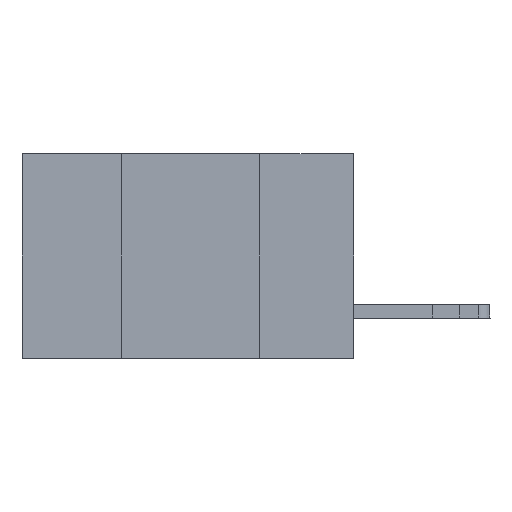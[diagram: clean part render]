
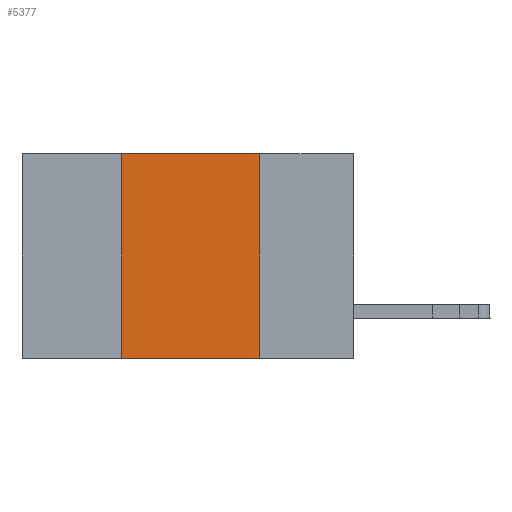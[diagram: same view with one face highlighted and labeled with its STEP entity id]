
A CAD part, left-side view. The second image highlights one B-rep face of the part: STEP entity #5377.
In plain terms, the highlighted planar face has unit normal (-1, 0, 0).
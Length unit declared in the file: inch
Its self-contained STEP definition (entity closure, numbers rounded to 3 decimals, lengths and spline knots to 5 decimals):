
#394 = VERTEX_POINT ( 'NONE', #6386 ) ;
#1948 = DIRECTION ( 'NONE',  ( 0., 0., -1. ) ) ;
#2194 = VERTEX_POINT ( 'NONE', #29420 ) ;
#3750 = CARTESIAN_POINT ( 'NONE',  ( 0., 0.6, -0.37 ) ) ;
#5377 = ADVANCED_FACE ( 'NONE', ( #24459 ), #15068, .F. ) ;
#5872 = VERTEX_POINT ( 'NONE', #25013 ) ;
#6386 = CARTESIAN_POINT ( 'NONE',  ( 0., 0.42, 0. ) ) ;
#6483 = DIRECTION ( 'NONE',  ( 0., -1., 0. ) ) ;
#6911 = DIRECTION ( 'NONE',  ( 1., 0., 0. ) ) ;
#7317 = CARTESIAN_POINT ( 'NONE',  ( 0., 0.17, 0. ) ) ;
#8722 = AXIS2_PLACEMENT_3D ( 'NONE', #23239, #6911, #25847 ) ;
#8817 = DIRECTION ( 'NONE',  ( 0., -1., 0. ) ) ;
#9220 = ORIENTED_EDGE ( 'NONE', *, *, #28491, .F. ) ;
#10951 = ORIENTED_EDGE ( 'NONE', *, *, #16478, .F. ) ;
#15068 = PLANE ( 'NONE',  #8722 ) ;
#15737 = EDGE_LOOP ( 'NONE', ( #9220, #10951, #18213, #32232 ) ) ;
#16478 = EDGE_CURVE ( 'NONE', #394, #24545, #31373, .T. ) ;
#17308 = CARTESIAN_POINT ( 'NONE',  ( 0., 0.17, 0. ) ) ;
#17313 = VECTOR ( 'NONE', #8817, 39.37008 ) ;
#18213 = ORIENTED_EDGE ( 'NONE', *, *, #24857, .F. ) ;
#19241 = VECTOR ( 'NONE', #6483, 39.37008 ) ;
#19705 = CARTESIAN_POINT ( 'NONE',  ( 0., 0.6, 0. ) ) ;
#22468 = VECTOR ( 'NONE', #1948, 39.37008 ) ;
#22738 = VECTOR ( 'NONE', #23661, 39.37008 ) ;
#23239 = CARTESIAN_POINT ( 'NONE',  ( 0., 0.6, 0. ) ) ;
#23661 = DIRECTION ( 'NONE',  ( 0., 0., 1. ) ) ;
#24459 = FACE_OUTER_BOUND ( 'NONE', #15737, .T. ) ;
#24545 = VERTEX_POINT ( 'NONE', #17308 ) ;
#24857 = EDGE_CURVE ( 'NONE', #2194, #394, #29676, .T. ) ;
#25013 = CARTESIAN_POINT ( 'NONE',  ( 0., 0.17, -0.37 ) ) ;
#25847 = DIRECTION ( 'NONE',  ( 0., 0., -1. ) ) ;
#28491 = EDGE_CURVE ( 'NONE', #24545, #5872, #29422, .T. ) ;
#29420 = CARTESIAN_POINT ( 'NONE',  ( 0., 0.42, -0.37 ) ) ;
#29422 = LINE ( 'NONE', #7317, #22468 ) ;
#29676 = LINE ( 'NONE', #31398, #22738 ) ;
#31373 = LINE ( 'NONE', #19705, #17313 ) ;
#31398 = CARTESIAN_POINT ( 'NONE',  ( 0., 0.42, 0. ) ) ;
#31930 = EDGE_CURVE ( 'NONE', #2194, #5872, #34017, .T. ) ;
#32232 = ORIENTED_EDGE ( 'NONE', *, *, #31930, .T. ) ;
#34017 = LINE ( 'NONE', #3750, #19241 ) ;
